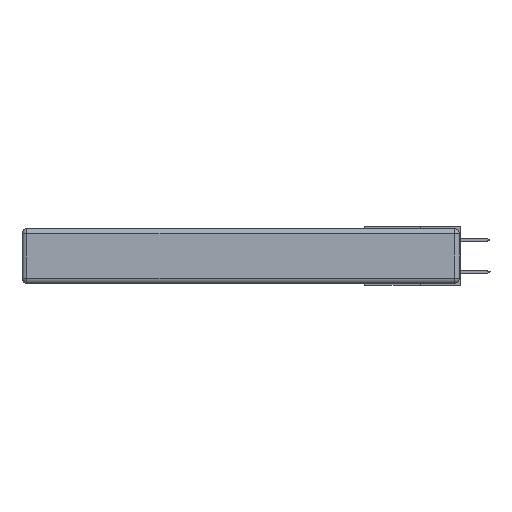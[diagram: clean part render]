
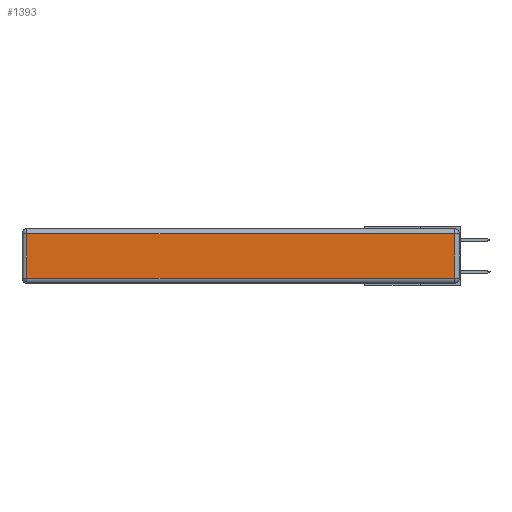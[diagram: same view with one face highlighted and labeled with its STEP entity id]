
A CAD part, left-side view. The second image highlights one B-rep face of the part: STEP entity #1393.
In plain terms, the highlighted planar face has unit normal (-1, 0, 0).
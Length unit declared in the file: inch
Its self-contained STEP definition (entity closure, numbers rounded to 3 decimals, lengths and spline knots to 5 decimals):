
#145 = DIRECTION ( 'NONE',  ( 0., 0., 1. ) ) ;
#307 = VECTOR ( 'NONE', #1940, 39.37008 ) ;
#999 = LINE ( 'NONE', #15058, #7345 ) ;
#1249 = PLANE ( 'NONE',  #12492 ) ;
#1393 = ADVANCED_FACE ( 'NONE', ( #4078 ), #1249, .T. ) ;
#1408 = ORIENTED_EDGE ( 'NONE', *, *, #13275, .T. ) ;
#1940 = DIRECTION ( 'NONE',  ( 0., -1., 0. ) ) ;
#2081 = CARTESIAN_POINT ( 'NONE',  ( 0., 0.03, -0.03 ) ) ;
#2416 = VERTEX_POINT ( 'NONE', #5486 ) ;
#4078 = FACE_OUTER_BOUND ( 'NONE', #13897, .T. ) ;
#4154 = ORIENTED_EDGE ( 'NONE', *, *, #11125, .T. ) ;
#4164 = DIRECTION ( 'NONE',  ( 0., 0., -1. ) ) ;
#4711 = DIRECTION ( 'NONE',  ( -1., 0., 0. ) ) ;
#5009 = LINE ( 'NONE', #15534, #14137 ) ;
#5486 = CARTESIAN_POINT ( 'NONE',  ( 0., 2.72, -0.313 ) ) ;
#7004 = CARTESIAN_POINT ( 'NONE',  ( 0., 0.03, -0.313 ) ) ;
#7007 = VERTEX_POINT ( 'NONE', #14982 ) ;
#7044 = ORIENTED_EDGE ( 'NONE', *, *, #12904, .T. ) ;
#7056 = LINE ( 'NONE', #10745, #307 ) ;
#7345 = VECTOR ( 'NONE', #145, 39.37008 ) ;
#7518 = ORIENTED_EDGE ( 'NONE', *, *, #15984, .T. ) ;
#8426 = DIRECTION ( 'NONE',  ( 0., 0., 1. ) ) ;
#9942 = DIRECTION ( 'NONE',  ( 0., 1., 0. ) ) ;
#10167 = VERTEX_POINT ( 'NONE', #2081 ) ;
#10745 = CARTESIAN_POINT ( 'NONE',  ( 0., 0., -0.313 ) ) ;
#11125 = EDGE_CURVE ( 'NONE', #7007, #2416, #5009, .T. ) ;
#12492 = AXIS2_PLACEMENT_3D ( 'NONE', #14706, #4711, #8426 ) ;
#12904 = EDGE_CURVE ( 'NONE', #10167, #7007, #14864, .T. ) ;
#13275 = EDGE_CURVE ( 'NONE', #2416, #15778, #7056, .T. ) ;
#13897 = EDGE_LOOP ( 'NONE', ( #1408, #7518, #7044, #4154 ) ) ;
#14137 = VECTOR ( 'NONE', #4164, 39.37008 ) ;
#14706 = CARTESIAN_POINT ( 'NONE',  ( 0., 0., -0.343 ) ) ;
#14864 = LINE ( 'NONE', #15118, #15470 ) ;
#14982 = CARTESIAN_POINT ( 'NONE',  ( 0., 2.72, -0.03 ) ) ;
#15058 = CARTESIAN_POINT ( 'NONE',  ( 0., 0.03, -0.343 ) ) ;
#15118 = CARTESIAN_POINT ( 'NONE',  ( 0., 2.75, -0.03 ) ) ;
#15470 = VECTOR ( 'NONE', #9942, 39.37008 ) ;
#15534 = CARTESIAN_POINT ( 'NONE',  ( 0., 2.72, -0.343 ) ) ;
#15778 = VERTEX_POINT ( 'NONE', #7004 ) ;
#15984 = EDGE_CURVE ( 'NONE', #15778, #10167, #999, .T. ) ;
